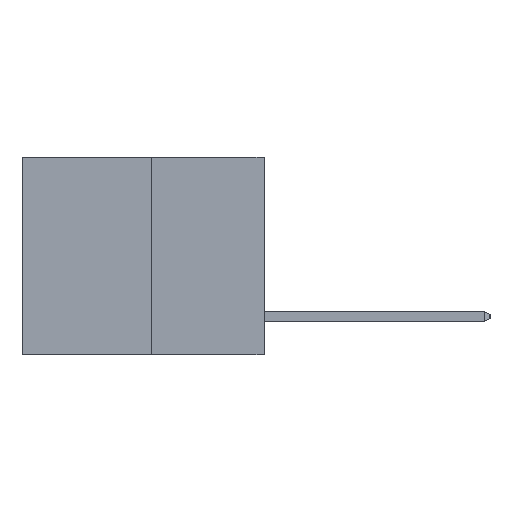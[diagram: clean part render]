
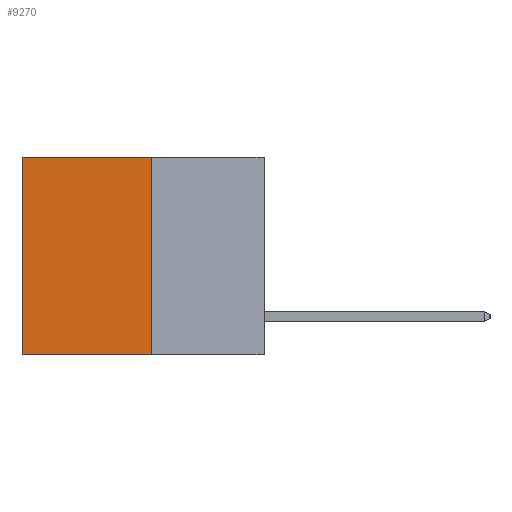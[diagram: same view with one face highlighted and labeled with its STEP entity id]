
A CAD part, left-side view. The second image highlights one B-rep face of the part: STEP entity #9270.
In plain terms, the highlighted planar face has unit normal (-1, 0, 0).
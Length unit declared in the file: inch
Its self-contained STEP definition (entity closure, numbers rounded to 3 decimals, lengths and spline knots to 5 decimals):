
#699 = VERTEX_POINT ( 'NONE', #7935 ) ;
#1835 = VECTOR ( 'NONE', #11036, 39.37008 ) ;
#2259 = LINE ( 'NONE', #8654, #12560 ) ;
#2586 = LINE ( 'NONE', #7538, #1835 ) ;
#2712 = CARTESIAN_POINT ( 'NONE',  ( 0.3165, 0.28, -0.49 ) ) ;
#3266 = CARTESIAN_POINT ( 'NONE',  ( 0.3165, 0.6, 0. ) ) ;
#3400 = FACE_OUTER_BOUND ( 'NONE', #7610, .T. ) ;
#3822 = CARTESIAN_POINT ( 'NONE',  ( 0.3165, 0.28, -0.49 ) ) ;
#4841 = CARTESIAN_POINT ( 'NONE',  ( 0.3165, 0.28, 0. ) ) ;
#5308 = ORIENTED_EDGE ( 'NONE', *, *, #10406, .F. ) ;
#5694 = VECTOR ( 'NONE', #9808, 39.37008 ) ;
#5717 = EDGE_CURVE ( 'NONE', #7041, #699, #12039, .T. ) ;
#5788 = ORIENTED_EDGE ( 'NONE', *, *, #10673, .T. ) ;
#6292 = PLANE ( 'NONE',  #11812 ) ;
#6923 = EDGE_CURVE ( 'NONE', #9902, #12923, #2259, .T. ) ;
#7041 = VERTEX_POINT ( 'NONE', #13039 ) ;
#7193 = DIRECTION ( 'NONE',  ( 0., 0., -1. ) ) ;
#7511 = DIRECTION ( 'NONE',  ( 0., 0., -1. ) ) ;
#7538 = CARTESIAN_POINT ( 'NONE',  ( 0.3165, 0.28, -0.49 ) ) ;
#7610 = EDGE_LOOP ( 'NONE', ( #5788, #10319, #5308, #10857 ) ) ;
#7739 = LINE ( 'NONE', #8175, #13370 ) ;
#7935 = CARTESIAN_POINT ( 'NONE',  ( 0.3165, 0.6, -0.49 ) ) ;
#8175 = CARTESIAN_POINT ( 'NONE',  ( 0.3165, 0.6, -0.49 ) ) ;
#8654 = CARTESIAN_POINT ( 'NONE',  ( 0.3165, 0.28, 0. ) ) ;
#8865 = DIRECTION ( 'NONE',  ( 1., 0., 0. ) ) ;
#9270 = ADVANCED_FACE ( 'NONE', ( #3400 ), #6292, .F. ) ;
#9808 = DIRECTION ( 'NONE',  ( 0., 1., 0. ) ) ;
#9902 = VERTEX_POINT ( 'NONE', #4841 ) ;
#9958 = DIRECTION ( 'NONE',  ( 0., 1., 0. ) ) ;
#10319 = ORIENTED_EDGE ( 'NONE', *, *, #5717, .F. ) ;
#10406 = EDGE_CURVE ( 'NONE', #9902, #7041, #2586, .T. ) ;
#10673 = EDGE_CURVE ( 'NONE', #12923, #699, #7739, .T. ) ;
#10857 = ORIENTED_EDGE ( 'NONE', *, *, #6923, .T. ) ;
#11036 = DIRECTION ( 'NONE',  ( 0., 0., -1. ) ) ;
#11812 = AXIS2_PLACEMENT_3D ( 'NONE', #2712, #8865, #7511 ) ;
#12039 = LINE ( 'NONE', #3822, #5694 ) ;
#12560 = VECTOR ( 'NONE', #9958, 39.37008 ) ;
#12923 = VERTEX_POINT ( 'NONE', #3266 ) ;
#13039 = CARTESIAN_POINT ( 'NONE',  ( 0.3165, 0.28, -0.49 ) ) ;
#13370 = VECTOR ( 'NONE', #7193, 39.37008 ) ;
